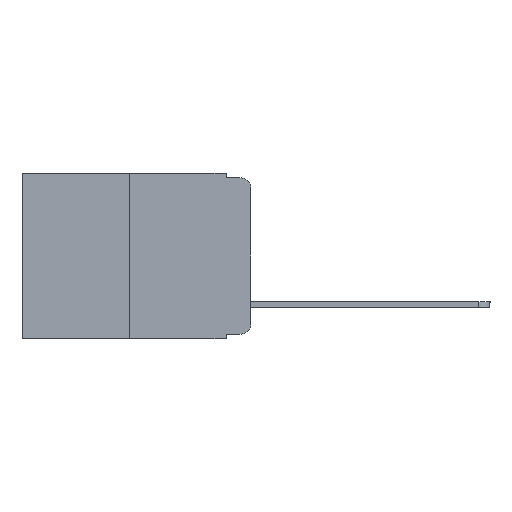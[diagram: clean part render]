
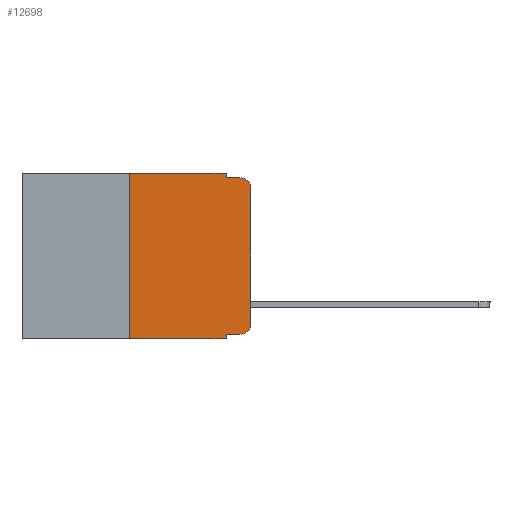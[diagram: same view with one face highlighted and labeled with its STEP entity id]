
A CAD part, left-side view. The second image highlights one B-rep face of the part: STEP entity #12698.
In plain terms, the highlighted planar face has unit normal (-1, 0, 0).
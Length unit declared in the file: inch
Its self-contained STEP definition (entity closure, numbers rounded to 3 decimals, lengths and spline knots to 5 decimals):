
#30 = VECTOR ( 'NONE', #18721, 39.37008 ) ;
#322 = VERTEX_POINT ( 'NONE', #3838 ) ;
#367 = EDGE_CURVE ( 'NONE', #5836, #322, #23189, .T. ) ;
#961 = EDGE_CURVE ( 'NONE', #2071, #24593, #13141, .T. ) ;
#1167 = CARTESIAN_POINT ( 'NONE',  ( 0., 0.473, -0.343 ) ) ;
#1621 = EDGE_CURVE ( 'NONE', #21993, #7762, #15734, .T. ) ;
#1642 = VERTEX_POINT ( 'NONE', #6222 ) ;
#2071 = VERTEX_POINT ( 'NONE', #8937 ) ;
#2205 = DIRECTION ( 'NONE',  ( 0., 0., 1. ) ) ;
#2417 = CARTESIAN_POINT ( 'NONE',  ( 0., 0.051, -0.333 ) ) ;
#2878 = ORIENTED_EDGE ( 'NONE', *, *, #23249, .F. ) ;
#2883 = DIRECTION ( 'NONE',  ( 1., 0., 0. ) ) ;
#2986 = DIRECTION ( 'NONE',  ( 0., 0., -1. ) ) ;
#3232 = EDGE_CURVE ( 'NONE', #1642, #5836, #20361, .T. ) ;
#3838 = CARTESIAN_POINT ( 'NONE',  ( 0., 0., -0.03 ) ) ;
#3910 = ORIENTED_EDGE ( 'NONE', *, *, #367, .T. ) ;
#3990 = CARTESIAN_POINT ( 'NONE',  ( 0., 0.051, -0.01 ) ) ;
#4196 = DIRECTION ( 'NONE',  ( 0., 0., 1. ) ) ;
#4347 = ORIENTED_EDGE ( 'NONE', *, *, #1621, .F. ) ;
#4390 = CARTESIAN_POINT ( 'NONE',  ( 0., 0.473, 0. ) ) ;
#4601 = CARTESIAN_POINT ( 'NONE',  ( 0., 0.473, 0. ) ) ;
#5836 = VERTEX_POINT ( 'NONE', #19495 ) ;
#6058 = LINE ( 'NONE', #11554, #6130 ) ;
#6130 = VECTOR ( 'NONE', #4196, 39.37008 ) ;
#6222 = CARTESIAN_POINT ( 'NONE',  ( 0., 0.02, -0.333 ) ) ;
#6267 = DIRECTION ( 'NONE',  ( 0., -1., 0. ) ) ;
#6906 = DIRECTION ( 'NONE',  ( 0., -1., 0. ) ) ;
#6956 = VECTOR ( 'NONE', #10869, 39.37008 ) ;
#7301 = ORIENTED_EDGE ( 'NONE', *, *, #8530, .F. ) ;
#7731 = ORIENTED_EDGE ( 'NONE', *, *, #17174, .F. ) ;
#7762 = VERTEX_POINT ( 'NONE', #17975 ) ;
#7846 = VECTOR ( 'NONE', #6906, 39.37008 ) ;
#8003 = EDGE_CURVE ( 'NONE', #2071, #21993, #6058, .T. ) ;
#8431 = CARTESIAN_POINT ( 'NONE',  ( 0., 0.02, -0.313 ) ) ;
#8530 = EDGE_CURVE ( 'NONE', #7762, #22976, #16252, .T. ) ;
#8809 = VERTEX_POINT ( 'NONE', #19247 ) ;
#8937 = CARTESIAN_POINT ( 'NONE',  ( 0., 0.25, -0.343 ) ) ;
#9060 = ORIENTED_EDGE ( 'NONE', *, *, #961, .T. ) ;
#9888 = ORIENTED_EDGE ( 'NONE', *, *, #3232, .T. ) ;
#10198 = DIRECTION ( 'NONE',  ( 0., 0., -1. ) ) ;
#10511 = DIRECTION ( 'NONE',  ( 0., 0., -1. ) ) ;
#10869 = DIRECTION ( 'NONE',  ( 0., 0., -1. ) ) ;
#11554 = CARTESIAN_POINT ( 'NONE',  ( 0., 0.25, 0. ) ) ;
#11564 = EDGE_CURVE ( 'NONE', #16321, #1642, #17912, .T. ) ;
#12315 = DIRECTION ( 'NONE',  ( -1., 0., 0. ) ) ;
#12365 = AXIS2_PLACEMENT_3D ( 'NONE', #8431, #12315, #10198 ) ;
#12414 = CARTESIAN_POINT ( 'NONE',  ( 0., 0.02, -0.03 ) ) ;
#12698 = ADVANCED_FACE ( 'NONE', ( #14000 ), #18147, .F. ) ;
#12961 = CARTESIAN_POINT ( 'NONE',  ( 0., 0.051, -0.343 ) ) ;
#13008 = CARTESIAN_POINT ( 'NONE',  ( 0., 0.051, -0.333 ) ) ;
#13141 = LINE ( 'NONE', #1167, #7846 ) ;
#13423 = ORIENTED_EDGE ( 'NONE', *, *, #19308, .T. ) ;
#13528 = ORIENTED_EDGE ( 'NONE', *, *, #8003, .F. ) ;
#13727 = DIRECTION ( 'NONE',  ( 0., -1., 0. ) ) ;
#14000 = FACE_OUTER_BOUND ( 'NONE', #23831, .T. ) ;
#14837 = ORIENTED_EDGE ( 'NONE', *, *, #11564, .T. ) ;
#15460 = CIRCLE ( 'NONE', #16653, 0.02 ) ;
#15734 = LINE ( 'NONE', #4601, #23040 ) ;
#16252 = LINE ( 'NONE', #20004, #6956 ) ;
#16321 = VERTEX_POINT ( 'NONE', #13008 ) ;
#16653 = AXIS2_PLACEMENT_3D ( 'NONE', #12414, #20062, #19557 ) ;
#17174 = EDGE_CURVE ( 'NONE', #16321, #24593, #21965, .T. ) ;
#17912 = LINE ( 'NONE', #2417, #19258 ) ;
#17975 = CARTESIAN_POINT ( 'NONE',  ( 0., 0.051, 0. ) ) ;
#18124 = AXIS2_PLACEMENT_3D ( 'NONE', #4390, #2883, #10511 ) ;
#18147 = PLANE ( 'NONE',  #18124 ) ;
#18721 = DIRECTION ( 'NONE',  ( 0., -1., 0. ) ) ;
#19247 = CARTESIAN_POINT ( 'NONE',  ( 0., 0.02, -0.01 ) ) ;
#19258 = VECTOR ( 'NONE', #6267, 39.37008 ) ;
#19308 = EDGE_CURVE ( 'NONE', #322, #8809, #15460, .T. ) ;
#19310 = LINE ( 'NONE', #21161, #30 ) ;
#19334 = CARTESIAN_POINT ( 'NONE',  ( 0., 0., 0. ) ) ;
#19495 = CARTESIAN_POINT ( 'NONE',  ( 0., 0., -0.313 ) ) ;
#19557 = DIRECTION ( 'NONE',  ( 0., 0., -1. ) ) ;
#20004 = CARTESIAN_POINT ( 'NONE',  ( 0., 0.051, 0. ) ) ;
#20062 = DIRECTION ( 'NONE',  ( -1., 0., 0. ) ) ;
#20120 = CARTESIAN_POINT ( 'NONE',  ( 0., 0.051, 0. ) ) ;
#20258 = VECTOR ( 'NONE', #2205, 39.37008 ) ;
#20361 = CIRCLE ( 'NONE', #12365, 0.02 ) ;
#20564 = VECTOR ( 'NONE', #2986, 39.37008 ) ;
#21161 = CARTESIAN_POINT ( 'NONE',  ( 0., 0.051, -0.01 ) ) ;
#21965 = LINE ( 'NONE', #20120, #20564 ) ;
#21993 = VERTEX_POINT ( 'NONE', #24302 ) ;
#22976 = VERTEX_POINT ( 'NONE', #3990 ) ;
#23040 = VECTOR ( 'NONE', #13727, 39.37008 ) ;
#23189 = LINE ( 'NONE', #19334, #20258 ) ;
#23249 = EDGE_CURVE ( 'NONE', #22976, #8809, #19310, .T. ) ;
#23831 = EDGE_LOOP ( 'NONE', ( #3910, #13423, #2878, #7301, #4347, #13528, #9060, #7731, #14837, #9888 ) ) ;
#24302 = CARTESIAN_POINT ( 'NONE',  ( 0., 0.25, 0. ) ) ;
#24593 = VERTEX_POINT ( 'NONE', #12961 ) ;
